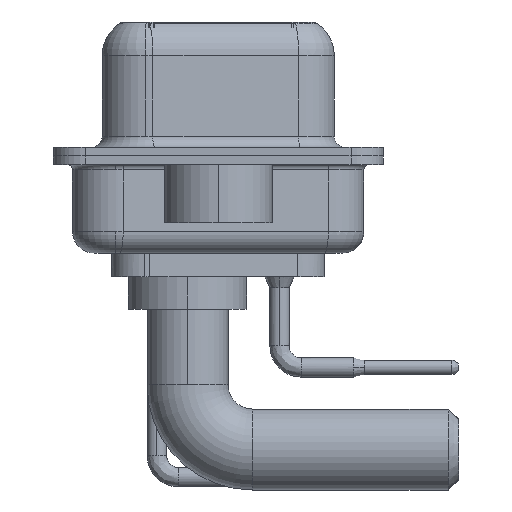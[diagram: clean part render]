
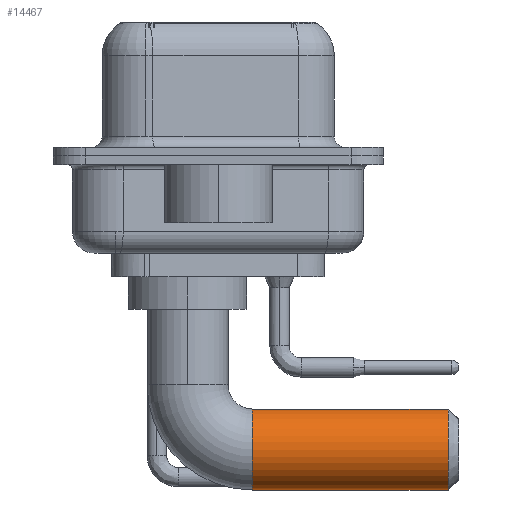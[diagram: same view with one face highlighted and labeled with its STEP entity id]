
A CAD part, left-side view. The second image highlights one B-rep face of the part: STEP entity #14467.
In plain terms, the highlighted cylindrical face has radius 1.875 mm (diameter 3.75 mm), a partial arc.
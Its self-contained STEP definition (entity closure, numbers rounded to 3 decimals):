
#151 = AXIS2_PLACEMENT_3D ( 'NONE', #14107, #17086, #29263 ) ;
#537 = CYLINDRICAL_SURFACE ( 'NONE', #4273, 1.875 ) ;
#702 = FACE_OUTER_BOUND ( 'NONE', #10254, .T. ) ;
#1013 = CARTESIAN_POINT ( 'NONE',  ( 0., -3., -6.5 ) ) ;
#1049 = EDGE_CURVE ( 'NONE', #3166, #3936, #9092, .T. ) ;
#1544 = CARTESIAN_POINT ( 'NONE',  ( 0., -3., -4.625 ) ) ;
#2154 = VECTOR ( 'NONE', #11399, 1000. ) ;
#2705 = EDGE_CURVE ( 'NONE', #28411, #29267, #6629, .T. ) ;
#3166 = VERTEX_POINT ( 'NONE', #31322 ) ;
#3833 = LINE ( 'NONE', #23906, #2154 ) ;
#3936 = VERTEX_POINT ( 'NONE', #25351 ) ;
#4020 = LINE ( 'NONE', #1544, #15394 ) ;
#4273 = AXIS2_PLACEMENT_3D ( 'NONE', #1013, #18453, #18134 ) ;
#6629 = CIRCLE ( 'NONE', #29212, 1.875 ) ;
#6754 = ORIENTED_EDGE ( 'NONE', *, *, #23980, .F. ) ;
#7384 = CARTESIAN_POINT ( 'NONE',  ( 0., -3., -4.625 ) ) ;
#8728 = ORIENTED_EDGE ( 'NONE', *, *, #1049, .T. ) ;
#9092 = CIRCLE ( 'NONE', #151, 1.875 ) ;
#10254 = EDGE_LOOP ( 'NONE', ( #6754, #29850, #14434, #8728 ) ) ;
#11399 = DIRECTION ( 'NONE',  ( 0., -1., 0. ) ) ;
#11478 = DIRECTION ( 'NONE',  ( 0., -1., 0. ) ) ;
#14107 = CARTESIAN_POINT ( 'NONE',  ( 0., -12.07, -6.5 ) ) ;
#14434 = ORIENTED_EDGE ( 'NONE', *, *, #31789, .T. ) ;
#14467 = ADVANCED_FACE ( 'NONE', ( #702 ), #537, .T. ) ;
#15394 = VECTOR ( 'NONE', #23435, 1000. ) ;
#16239 = DIRECTION ( 'NONE',  ( -1., 0., 0. ) ) ;
#17086 = DIRECTION ( 'NONE',  ( 0., 1., 0. ) ) ;
#18134 = DIRECTION ( 'NONE',  ( 0., 0., -1. ) ) ;
#18453 = DIRECTION ( 'NONE',  ( 0., -1., 0. ) ) ;
#18547 = CARTESIAN_POINT ( 'NONE',  ( 0., -3., -6.5 ) ) ;
#23435 = DIRECTION ( 'NONE',  ( 0., -1., 0. ) ) ;
#23906 = CARTESIAN_POINT ( 'NONE',  ( 0., -3., -8.375 ) ) ;
#23980 = EDGE_CURVE ( 'NONE', #28411, #3936, #4020, .T. ) ;
#25351 = CARTESIAN_POINT ( 'NONE',  ( 0., -12.07, -4.625 ) ) ;
#27999 = CARTESIAN_POINT ( 'NONE',  ( 0., -3., -8.375 ) ) ;
#28411 = VERTEX_POINT ( 'NONE', #7384 ) ;
#29212 = AXIS2_PLACEMENT_3D ( 'NONE', #18547, #11478, #16239 ) ;
#29263 = DIRECTION ( 'NONE',  ( 0., 0., -1. ) ) ;
#29267 = VERTEX_POINT ( 'NONE', #27999 ) ;
#29850 = ORIENTED_EDGE ( 'NONE', *, *, #2705, .T. ) ;
#31322 = CARTESIAN_POINT ( 'NONE',  ( 0., -12.07, -8.375 ) ) ;
#31789 = EDGE_CURVE ( 'NONE', #29267, #3166, #3833, .T. ) ;
